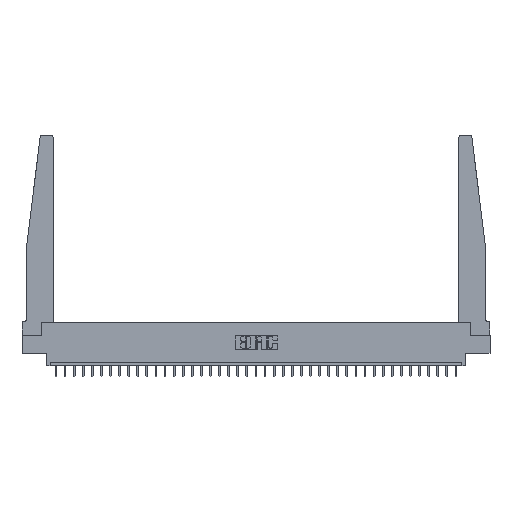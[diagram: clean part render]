
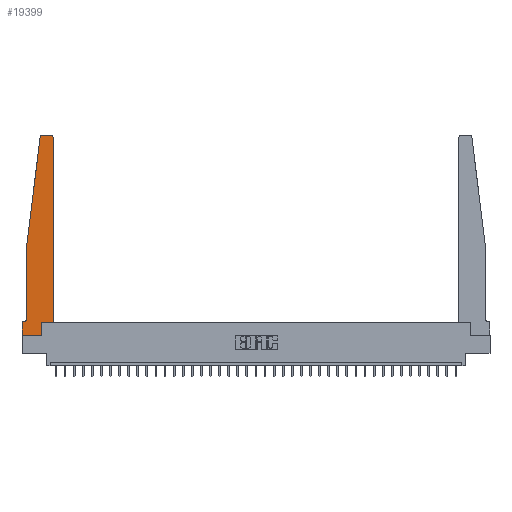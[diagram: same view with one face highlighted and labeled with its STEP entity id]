
A CAD part, top view. The second image highlights one B-rep face of the part: STEP entity #19399.
In plain terms, the highlighted planar face has unit normal (0, 0, 1).
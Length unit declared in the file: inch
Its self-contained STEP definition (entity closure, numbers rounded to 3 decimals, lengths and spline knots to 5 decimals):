
#14 = DIRECTION ( 'NONE',  ( 1., 0., 0. ) ) ;
#743 = CARTESIAN_POINT ( 'NONE',  ( 0.2605, 0., 0.37 ) ) ;
#1300 = CARTESIAN_POINT ( 'NONE',  ( 0.065, 1.25, 0.37 ) ) ;
#2097 = ORIENTED_EDGE ( 'NONE', *, *, #29227, .T. ) ;
#2165 = CARTESIAN_POINT ( 'NONE',  ( 0., 0., 0.37 ) ) ;
#2209 = VECTOR ( 'NONE', #31914, 39.37008 ) ;
#2368 = CARTESIAN_POINT ( 'NONE',  ( 0.425, 0.18, 0.37 ) ) ;
#2407 = CIRCLE ( 'NONE', #12482, 0.03 ) ;
#2440 = EDGE_CURVE ( 'NONE', #8812, #31687, #21071, .T. ) ;
#2605 = CARTESIAN_POINT ( 'NONE',  ( 0.27653, 2.75, 0.37 ) ) ;
#2912 = AXIS2_PLACEMENT_3D ( 'NONE', #29899, #26903, #27552 ) ;
#2960 = ORIENTED_EDGE ( 'NONE', *, *, #7725, .T. ) ;
#2970 = LINE ( 'NONE', #13078, #20984 ) ;
#3129 = CARTESIAN_POINT ( 'NONE',  ( 0.065, 0.1875, 0.37 ) ) ;
#3288 = ORIENTED_EDGE ( 'NONE', *, *, #24631, .T. ) ;
#3459 = CARTESIAN_POINT ( 'NONE',  ( 0., 0.1875, 0.37 ) ) ;
#4956 = DIRECTION ( 'NONE',  ( 0., 0., 1. ) ) ;
#4976 = DIRECTION ( 'NONE',  ( 1., 0., 0. ) ) ;
#5008 = ORIENTED_EDGE ( 'NONE', *, *, #16012, .T. ) ;
#5010 = ORIENTED_EDGE ( 'NONE', *, *, #17253, .T. ) ;
#5413 = CARTESIAN_POINT ( 'NONE',  ( 0.25, 2.75, 0.37 ) ) ;
#5599 = ORIENTED_EDGE ( 'NONE', *, *, #2440, .T. ) ;
#6068 = VECTOR ( 'NONE', #11480, 39.37008 ) ;
#6453 = CARTESIAN_POINT ( 'NONE',  ( 0.2605, 0.18, 0.37 ) ) ;
#6469 = DIRECTION ( 'NONE',  ( 0., -1., 0. ) ) ;
#7725 = EDGE_CURVE ( 'NONE', #31845, #18223, #32051, .T. ) ;
#7760 = CARTESIAN_POINT ( 'NONE',  ( 0.24675, 2.72367, 0.37 ) ) ;
#7807 = DIRECTION ( 'NONE',  ( -1., 0., 0. ) ) ;
#8812 = VERTEX_POINT ( 'NONE', #28443 ) ;
#8900 = VECTOR ( 'NONE', #11728, 39.37008 ) ;
#9261 = DIRECTION ( 'NONE',  ( 0., 1., 0. ) ) ;
#9475 = CARTESIAN_POINT ( 'NONE',  ( 0.065, 0.2375, 0.37 ) ) ;
#9973 = DIRECTION ( 'NONE',  ( 0., 0., 1. ) ) ;
#10004 = EDGE_LOOP ( 'NONE', ( #2097, #5008, #23580, #5599, #17073, #3288, #14150, #21597, #28770, #5010, #2960, #24514 ) ) ;
#10077 = CARTESIAN_POINT ( 'NONE',  ( 0.395, 2.75, 0.37 ) ) ;
#10598 = FACE_OUTER_BOUND ( 'NONE', #10004, .T. ) ;
#11159 = EDGE_CURVE ( 'NONE', #13241, #11630, #22802, .T. ) ;
#11480 = DIRECTION ( 'NONE',  ( 1., 0., 0. ) ) ;
#11540 = VERTEX_POINT ( 'NONE', #10077 ) ;
#11574 = CARTESIAN_POINT ( 'NONE',  ( 0.015, 0.1875, 0.37 ) ) ;
#11630 = VERTEX_POINT ( 'NONE', #743 ) ;
#11728 = DIRECTION ( 'NONE',  ( 0., 1., 0. ) ) ;
#12037 = CARTESIAN_POINT ( 'NONE',  ( 0.425, 0.18, 0.37 ) ) ;
#12427 = CIRCLE ( 'NONE', #2912, 0.05 ) ;
#12482 = AXIS2_PLACEMENT_3D ( 'NONE', #32745, #20094, #4976 ) ;
#13078 = CARTESIAN_POINT ( 'NONE',  ( 0., 0., 0.37 ) ) ;
#13241 = VERTEX_POINT ( 'NONE', #2165 ) ;
#14150 = ORIENTED_EDGE ( 'NONE', *, *, #25959, .T. ) ;
#14595 = CARTESIAN_POINT ( 'NONE',  ( 0.425, 0.18, 0.37 ) ) ;
#15084 = DIRECTION ( 'NONE',  ( 1., 0., 0. ) ) ;
#15527 = DIRECTION ( 'NONE',  ( -1., 0., 0. ) ) ;
#16012 = EDGE_CURVE ( 'NONE', #32406, #18498, #26436, .T. ) ;
#16493 = VECTOR ( 'NONE', #9261, 39.37008 ) ;
#17073 = ORIENTED_EDGE ( 'NONE', *, *, #24971, .T. ) ;
#17253 = EDGE_CURVE ( 'NONE', #24719, #31845, #25166, .T. ) ;
#17450 = DIRECTION ( 'NONE',  ( 1., 0., 0. ) ) ;
#18223 = VERTEX_POINT ( 'NONE', #21392 ) ;
#18314 = VERTEX_POINT ( 'NONE', #11574 ) ;
#18498 = VERTEX_POINT ( 'NONE', #7760 ) ;
#19399 = ADVANCED_FACE ( 'NONE', ( #10598 ), #25749, .T. ) ;
#20094 = DIRECTION ( 'NONE',  ( 0., 0., 1. ) ) ;
#20984 = VECTOR ( 'NONE', #23258, 39.37008 ) ;
#21071 = LINE ( 'NONE', #1300, #31746 ) ;
#21392 = CARTESIAN_POINT ( 'NONE',  ( 0.425, 2.72, 0.37 ) ) ;
#21597 = ORIENTED_EDGE ( 'NONE', *, *, #11159, .T. ) ;
#22179 = VERTEX_POINT ( 'NONE', #3459 ) ;
#22218 = EDGE_CURVE ( 'NONE', #18498, #8812, #31434, .T. ) ;
#22543 = LINE ( 'NONE', #5413, #24584 ) ;
#22802 = LINE ( 'NONE', #27311, #30460 ) ;
#23239 = CARTESIAN_POINT ( 'NONE',  ( 0., 0.1875, 0.37 ) ) ;
#23258 = DIRECTION ( 'NONE',  ( 0., -1., 0. ) ) ;
#23580 = ORIENTED_EDGE ( 'NONE', *, *, #22218, .T. ) ;
#24380 = LINE ( 'NONE', #6453, #8900 ) ;
#24514 = ORIENTED_EDGE ( 'NONE', *, *, #25821, .T. ) ;
#24584 = VECTOR ( 'NONE', #15527, 39.37008 ) ;
#24631 = EDGE_CURVE ( 'NONE', #18314, #22179, #25916, .T. ) ;
#24719 = VERTEX_POINT ( 'NONE', #30428 ) ;
#24971 = EDGE_CURVE ( 'NONE', #31687, #18314, #12427, .T. ) ;
#25166 = LINE ( 'NONE', #2368, #6068 ) ;
#25187 = VECTOR ( 'NONE', #7807, 39.37008 ) ;
#25749 = PLANE ( 'NONE',  #30169 ) ;
#25821 = EDGE_CURVE ( 'NONE', #18223, #11540, #2407, .T. ) ;
#25916 = LINE ( 'NONE', #3129, #25187 ) ;
#25959 = EDGE_CURVE ( 'NONE', #22179, #13241, #2970, .T. ) ;
#26436 = CIRCLE ( 'NONE', #31764, 0.03 ) ;
#26903 = DIRECTION ( 'NONE',  ( 0., 0., -1. ) ) ;
#27311 = CARTESIAN_POINT ( 'NONE',  ( 0., 0., 0.37 ) ) ;
#27552 = DIRECTION ( 'NONE',  ( -1., 0., 0. ) ) ;
#28443 = CARTESIAN_POINT ( 'NONE',  ( 0.065, 1.25, 0.37 ) ) ;
#28770 = ORIENTED_EDGE ( 'NONE', *, *, #30824, .T. ) ;
#28912 = CARTESIAN_POINT ( 'NONE',  ( 0.065, 1.25, 0.37 ) ) ;
#29227 = EDGE_CURVE ( 'NONE', #11540, #32406, #22543, .T. ) ;
#29899 = CARTESIAN_POINT ( 'NONE',  ( 0.015, 0.2375, 0.37 ) ) ;
#30169 = AXIS2_PLACEMENT_3D ( 'NONE', #23239, #4956, #15084 ) ;
#30285 = CARTESIAN_POINT ( 'NONE',  ( 0.27653, 2.72, 0.37 ) ) ;
#30428 = CARTESIAN_POINT ( 'NONE',  ( 0.2605, 0.18, 0.37 ) ) ;
#30460 = VECTOR ( 'NONE', #14, 39.37008 ) ;
#30824 = EDGE_CURVE ( 'NONE', #11630, #24719, #24380, .T. ) ;
#31434 = LINE ( 'NONE', #28912, #2209 ) ;
#31687 = VERTEX_POINT ( 'NONE', #9475 ) ;
#31746 = VECTOR ( 'NONE', #6469, 39.37008 ) ;
#31764 = AXIS2_PLACEMENT_3D ( 'NONE', #30285, #9973, #17450 ) ;
#31845 = VERTEX_POINT ( 'NONE', #14595 ) ;
#31914 = DIRECTION ( 'NONE',  ( -0.122, -0.992, 0. ) ) ;
#32051 = LINE ( 'NONE', #12037, #16493 ) ;
#32406 = VERTEX_POINT ( 'NONE', #2605 ) ;
#32745 = CARTESIAN_POINT ( 'NONE',  ( 0.395, 2.72, 0.37 ) ) ;
